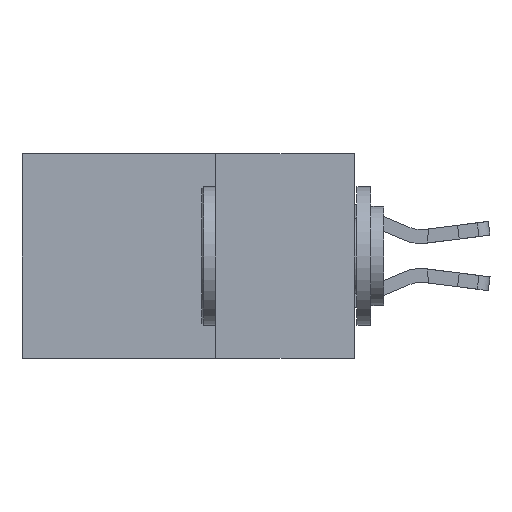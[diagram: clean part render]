
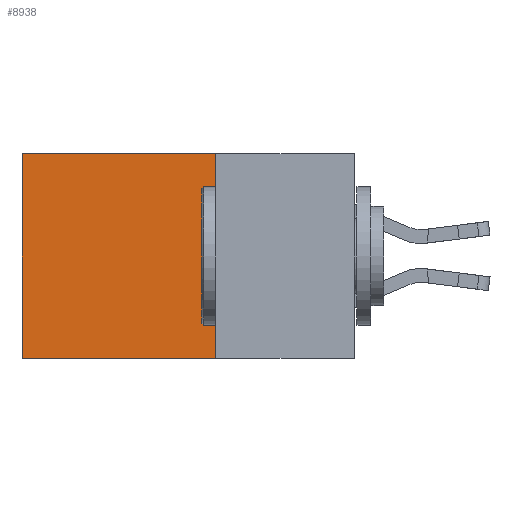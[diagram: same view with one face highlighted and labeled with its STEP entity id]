
A CAD part, left-side view. The second image highlights one B-rep face of the part: STEP entity #8938.
In plain terms, the highlighted planar face has unit normal (-1, 0, 0).
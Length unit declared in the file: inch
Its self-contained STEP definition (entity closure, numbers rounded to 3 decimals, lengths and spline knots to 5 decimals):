
#1331 = EDGE_CURVE ( 'NONE', #8840, #4601, #13881, .T. ) ;
#2203 = LINE ( 'NONE', #14317, #14954 ) ;
#2494 = ORIENTED_EDGE ( 'NONE', *, *, #15522, .F. ) ;
#3024 = DIRECTION ( 'NONE',  ( 0., 0., -1. ) ) ;
#4601 = VERTEX_POINT ( 'NONE', #20327 ) ;
#4654 = ORIENTED_EDGE ( 'NONE', *, *, #1331, .T. ) ;
#6279 = EDGE_CURVE ( 'NONE', #8840, #20130, #11834, .T. ) ;
#6501 = DIRECTION ( 'NONE',  ( 0., 1., 0. ) ) ;
#8346 = DIRECTION ( 'NONE',  ( 0., 0., -1. ) ) ;
#8840 = VERTEX_POINT ( 'NONE', #19453 ) ;
#8938 = ADVANCED_FACE ( 'NONE', ( #14796 ), #14873, .F. ) ;
#9046 = DIRECTION ( 'NONE',  ( 0., 1., 0. ) ) ;
#10344 = ORIENTED_EDGE ( 'NONE', *, *, #17658, .T. ) ;
#11352 = CARTESIAN_POINT ( 'NONE',  ( 0.2615, 0.25, -0.37 ) ) ;
#11834 = LINE ( 'NONE', #11352, #15652 ) ;
#12285 = CARTESIAN_POINT ( 'NONE',  ( 0.2615, 0.25, 0. ) ) ;
#12531 = ORIENTED_EDGE ( 'NONE', *, *, #6279, .F. ) ;
#13359 = VECTOR ( 'NONE', #9046, 39.37008 ) ;
#13881 = LINE ( 'NONE', #12285, #13359 ) ;
#14317 = CARTESIAN_POINT ( 'NONE',  ( 0.2615, 0.6, -0.37 ) ) ;
#14653 = AXIS2_PLACEMENT_3D ( 'NONE', #16487, #18126, #8346 ) ;
#14728 = CARTESIAN_POINT ( 'NONE',  ( 0.2615, 0.25, -0.37 ) ) ;
#14796 = FACE_OUTER_BOUND ( 'NONE', #15666, .T. ) ;
#14873 = PLANE ( 'NONE',  #14653 ) ;
#14954 = VECTOR ( 'NONE', #15936, 39.37008 ) ;
#15016 = CARTESIAN_POINT ( 'NONE',  ( 0.2615, 0.25, -0.37 ) ) ;
#15522 = EDGE_CURVE ( 'NONE', #20130, #19767, #17113, .T. ) ;
#15652 = VECTOR ( 'NONE', #3024, 39.37008 ) ;
#15666 = EDGE_LOOP ( 'NONE', ( #10344, #2494, #12531, #4654 ) ) ;
#15936 = DIRECTION ( 'NONE',  ( 0., 0., -1. ) ) ;
#16487 = CARTESIAN_POINT ( 'NONE',  ( 0.2615, 0.25, -0.37 ) ) ;
#17113 = LINE ( 'NONE', #14728, #20836 ) ;
#17362 = CARTESIAN_POINT ( 'NONE',  ( 0.2615, 0.6, -0.37 ) ) ;
#17658 = EDGE_CURVE ( 'NONE', #4601, #19767, #2203, .T. ) ;
#18126 = DIRECTION ( 'NONE',  ( 1., 0., 0. ) ) ;
#19453 = CARTESIAN_POINT ( 'NONE',  ( 0.2615, 0.25, 0. ) ) ;
#19767 = VERTEX_POINT ( 'NONE', #17362 ) ;
#20130 = VERTEX_POINT ( 'NONE', #15016 ) ;
#20327 = CARTESIAN_POINT ( 'NONE',  ( 0.2615, 0.6, 0. ) ) ;
#20836 = VECTOR ( 'NONE', #6501, 39.37008 ) ;
